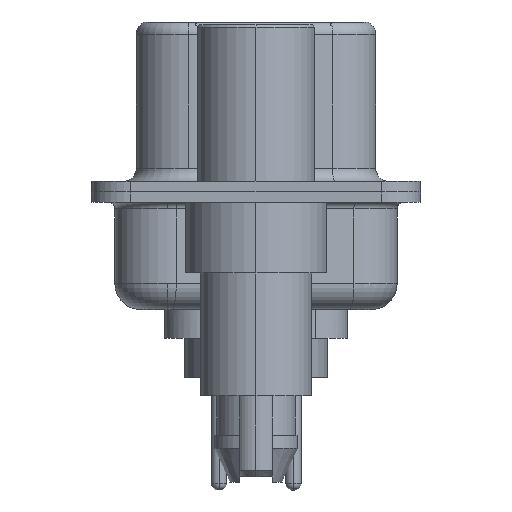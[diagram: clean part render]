
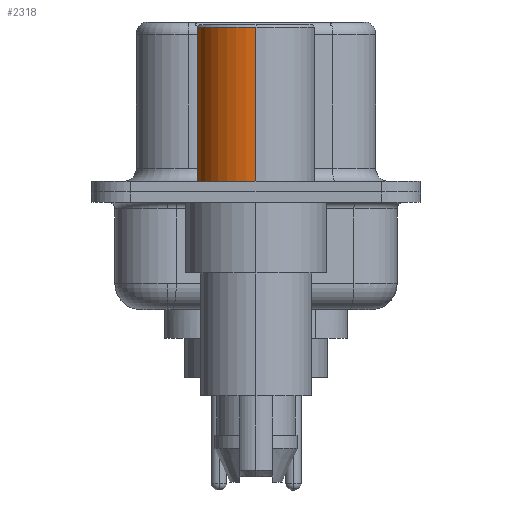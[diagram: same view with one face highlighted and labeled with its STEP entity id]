
A CAD part, left-side view. The second image highlights one B-rep face of the part: STEP entity #2318.
In plain terms, the highlighted cylindrical face has radius 2.25 mm (diameter 4.5 mm), a partial arc.
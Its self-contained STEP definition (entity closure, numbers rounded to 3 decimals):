
#919 = CYLINDRICAL_SURFACE ( 'NONE', #20733, 2.25 ) ;
#1116 = VECTOR ( 'NONE', #22380, 1000. ) ;
#1860 = VERTEX_POINT ( 'NONE', #17041 ) ;
#2318 = ADVANCED_FACE ( 'NONE', ( #7222 ), #919, .T. ) ;
#2332 = AXIS2_PLACEMENT_3D ( 'NONE', #2509, #9570, #9663 ) ;
#2509 = CARTESIAN_POINT ( 'NONE',  ( 0., 0., 6.3 ) ) ;
#2544 = EDGE_LOOP ( 'NONE', ( #26221, #12987, #11710, #22849 ) ) ;
#4517 = VERTEX_POINT ( 'NONE', #26186 ) ;
#5668 = DIRECTION ( 'NONE',  ( 1., 0., 0. ) ) ;
#6248 = EDGE_CURVE ( 'NONE', #22535, #4517, #8947, .T. ) ;
#7105 = DIRECTION ( 'NONE',  ( 0., 0., 1. ) ) ;
#7222 = FACE_OUTER_BOUND ( 'NONE', #2544, .T. ) ;
#8126 = CARTESIAN_POINT ( 'NONE',  ( 2.25, 0., 0.581 ) ) ;
#8272 = CARTESIAN_POINT ( 'NONE',  ( 2.25, 0., 6.3 ) ) ;
#8486 = AXIS2_PLACEMENT_3D ( 'NONE', #19329, #7105, #21417 ) ;
#8947 = CIRCLE ( 'NONE', #2332, 2.25 ) ;
#9262 = CARTESIAN_POINT ( 'NONE',  ( 0., 0., 0.581 ) ) ;
#9339 = LINE ( 'NONE', #19088, #23737 ) ;
#9570 = DIRECTION ( 'NONE',  ( 0., 0., 1. ) ) ;
#9663 = DIRECTION ( 'NONE',  ( 1., 0., 0. ) ) ;
#11710 = ORIENTED_EDGE ( 'NONE', *, *, #6248, .F. ) ;
#12987 = ORIENTED_EDGE ( 'NONE', *, *, #25673, .T. ) ;
#14848 = CIRCLE ( 'NONE', #8486, 2.25 ) ;
#16396 = LINE ( 'NONE', #8126, #1116 ) ;
#17041 = CARTESIAN_POINT ( 'NONE',  ( -2.25, 0., 0.4 ) ) ;
#18942 = EDGE_CURVE ( 'NONE', #21552, #1860, #14848, .T. ) ;
#19088 = CARTESIAN_POINT ( 'NONE',  ( -2.25, 0., 0.581 ) ) ;
#19174 = DIRECTION ( 'NONE',  ( 0., 0., 1. ) ) ;
#19329 = CARTESIAN_POINT ( 'NONE',  ( 0., 0., 0.4 ) ) ;
#19479 = CARTESIAN_POINT ( 'NONE',  ( 2.25, 0., 0.4 ) ) ;
#20070 = EDGE_CURVE ( 'NONE', #21552, #22535, #16396, .T. ) ;
#20733 = AXIS2_PLACEMENT_3D ( 'NONE', #9262, #23975, #5668 ) ;
#21417 = DIRECTION ( 'NONE',  ( 1., 0., 0. ) ) ;
#21552 = VERTEX_POINT ( 'NONE', #19479 ) ;
#22380 = DIRECTION ( 'NONE',  ( 0., 0., 1. ) ) ;
#22535 = VERTEX_POINT ( 'NONE', #8272 ) ;
#22849 = ORIENTED_EDGE ( 'NONE', *, *, #20070, .F. ) ;
#23737 = VECTOR ( 'NONE', #19174, 1000. ) ;
#23975 = DIRECTION ( 'NONE',  ( 0., 0., 1. ) ) ;
#25673 = EDGE_CURVE ( 'NONE', #1860, #4517, #9339, .T. ) ;
#26186 = CARTESIAN_POINT ( 'NONE',  ( -2.25, 0., 6.3 ) ) ;
#26221 = ORIENTED_EDGE ( 'NONE', *, *, #18942, .T. ) ;
